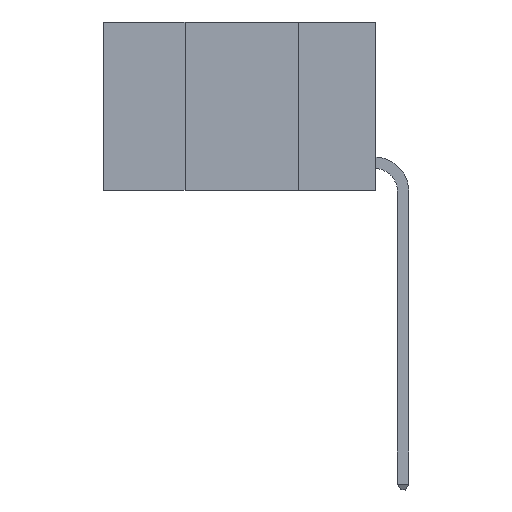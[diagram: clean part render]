
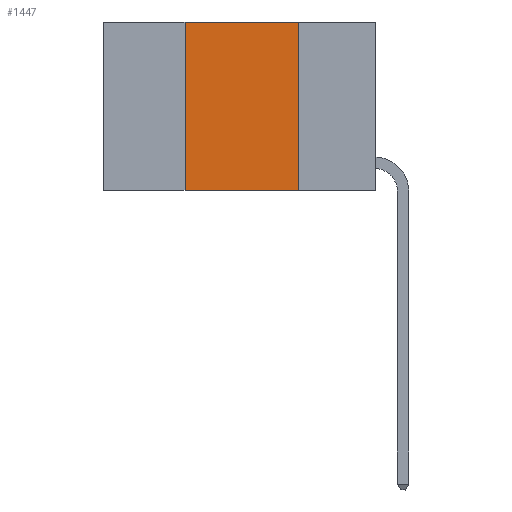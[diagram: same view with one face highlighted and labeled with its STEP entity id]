
A CAD part, left-side view. The second image highlights one B-rep face of the part: STEP entity #1447.
In plain terms, the highlighted planar face has unit normal (-1, 0, 0).
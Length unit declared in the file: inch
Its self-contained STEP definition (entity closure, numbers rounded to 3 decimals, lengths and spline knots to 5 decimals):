
#122 = LINE ( 'NONE', #942, #6940 ) ;
#779 = FACE_OUTER_BOUND ( 'NONE', #7800, .T. ) ;
#942 = CARTESIAN_POINT ( 'NONE',  ( 0., 0.6, 0. ) ) ;
#1054 = VERTEX_POINT ( 'NONE', #9311 ) ;
#1282 = CARTESIAN_POINT ( 'NONE',  ( 0., 0.42, -0.37 ) ) ;
#1447 = ADVANCED_FACE ( 'NONE', ( #779 ), #14954, .F. ) ;
#2575 = VERTEX_POINT ( 'NONE', #12739 ) ;
#2900 = DIRECTION ( 'NONE',  ( 0., -1., 0. ) ) ;
#5234 = EDGE_CURVE ( 'NONE', #18924, #2575, #7478, .T. ) ;
#5972 = DIRECTION ( 'NONE',  ( 0., 0., -1. ) ) ;
#6940 = VECTOR ( 'NONE', #13450, 39.37008 ) ;
#7478 = LINE ( 'NONE', #16467, #13142 ) ;
#7800 = EDGE_LOOP ( 'NONE', ( #21958, #11091, #15311, #16895 ) ) ;
#8509 = EDGE_CURVE ( 'NONE', #18729, #2575, #15505, .T. ) ;
#8773 = CARTESIAN_POINT ( 'NONE',  ( 0., 0.6, -0.37 ) ) ;
#9311 = CARTESIAN_POINT ( 'NONE',  ( 0., 0.42, 0. ) ) ;
#11091 = ORIENTED_EDGE ( 'NONE', *, *, #20632, .F. ) ;
#11692 = DIRECTION ( 'NONE',  ( 0., 0., 1. ) ) ;
#12739 = CARTESIAN_POINT ( 'NONE',  ( 0., 0.17, -0.37 ) ) ;
#13142 = VECTOR ( 'NONE', #14814, 39.37008 ) ;
#13450 = DIRECTION ( 'NONE',  ( 0., -1., 0. ) ) ;
#14814 = DIRECTION ( 'NONE',  ( 0., 0., -1. ) ) ;
#14954 = PLANE ( 'NONE',  #16036 ) ;
#15311 = ORIENTED_EDGE ( 'NONE', *, *, #17408, .F. ) ;
#15319 = CARTESIAN_POINT ( 'NONE',  ( 0., 0.42, 0. ) ) ;
#15505 = LINE ( 'NONE', #8773, #20519 ) ;
#16036 = AXIS2_PLACEMENT_3D ( 'NONE', #20532, #21080, #5972 ) ;
#16467 = CARTESIAN_POINT ( 'NONE',  ( 0., 0.17, 0. ) ) ;
#16895 = ORIENTED_EDGE ( 'NONE', *, *, #8509, .T. ) ;
#17408 = EDGE_CURVE ( 'NONE', #18729, #1054, #21015, .T. ) ;
#18729 = VERTEX_POINT ( 'NONE', #1282 ) ;
#18821 = CARTESIAN_POINT ( 'NONE',  ( 0., 0.17, 0. ) ) ;
#18924 = VERTEX_POINT ( 'NONE', #18821 ) ;
#20519 = VECTOR ( 'NONE', #2900, 39.37008 ) ;
#20532 = CARTESIAN_POINT ( 'NONE',  ( 0., 0.6, 0. ) ) ;
#20632 = EDGE_CURVE ( 'NONE', #1054, #18924, #122, .T. ) ;
#21015 = LINE ( 'NONE', #15319, #22335 ) ;
#21080 = DIRECTION ( 'NONE',  ( 1., 0., 0. ) ) ;
#21958 = ORIENTED_EDGE ( 'NONE', *, *, #5234, .F. ) ;
#22335 = VECTOR ( 'NONE', #11692, 39.37008 ) ;
